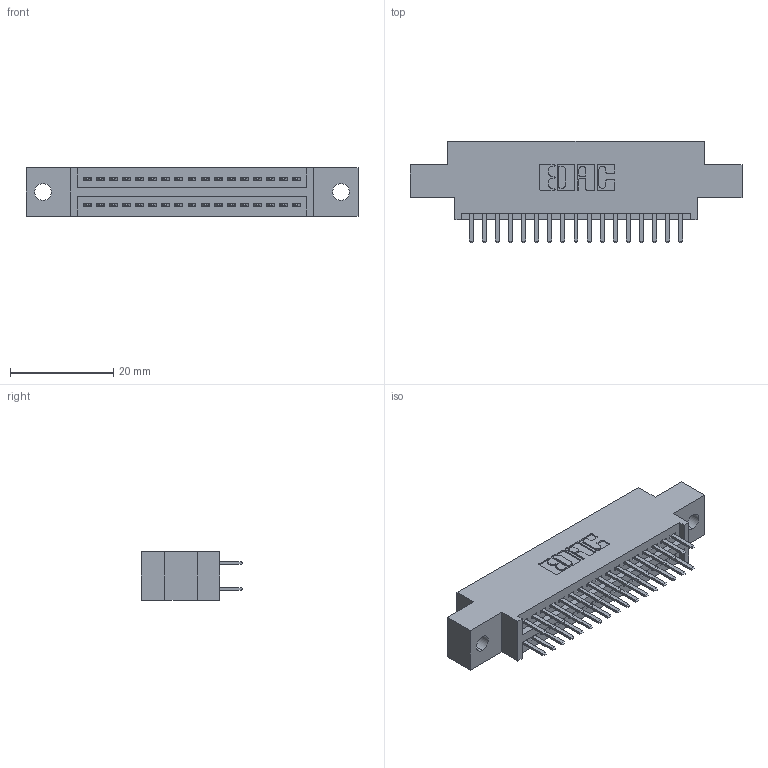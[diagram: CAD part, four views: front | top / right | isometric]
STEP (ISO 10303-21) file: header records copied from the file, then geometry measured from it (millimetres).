
FILE_DESCRIPTION (( 'STEP AP203' ), '1' );
FILE_NAME ('345-034-520-802.STEP', '2019-10-28T05:56:29', ( '' ), ( '' ), 'SwSTEP 2.0', 'SolidWorks 2016', '' );
FILE_SCHEMA (( 'CONFIG_CONTROL_DESIGN' ));
Length unit declared in the file: inch
Products named in the file (3): 345-292-001_345-293-120; 345 Part_0.170 Offset - 0.128 Dia; 345-034-520-802
Assembly tree (35 placements, depth 2):
  345-034-520-802
    345 Part_0.170 Offset - 0.128 Dia
    345-292-001_345-293-120  x34
Bounding box: 64.39 x 19.68 x 9.4 mm (x, y, z)
Volume: 5857.7 mm3; surface area: 8013.5 mm2
Topology: 35 solids, 35 shells, 1966 faces, 5691 edges, 3702 vertices
Faces by surface type: plane 1274, cylinder 692
Entity records: 16953 total; most frequent: CARTESIAN_POINT 2880, ORIENTED_EDGE 2802, DIRECTION 2557, EDGE_CURVE 1401, VECTOR 1197, LINE 1197, VERTEX_POINT 930, AXIS2_PLACEMENT_3D 680
